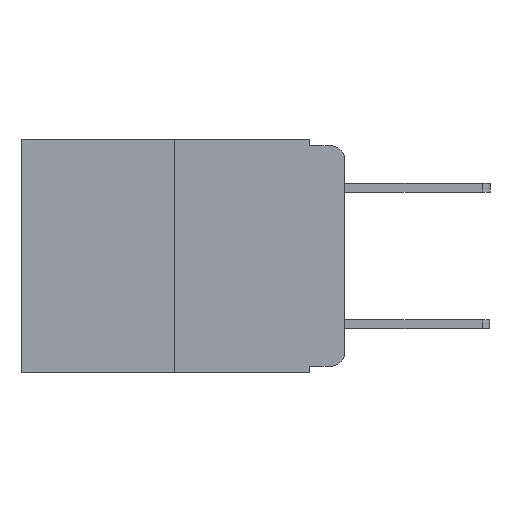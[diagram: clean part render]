
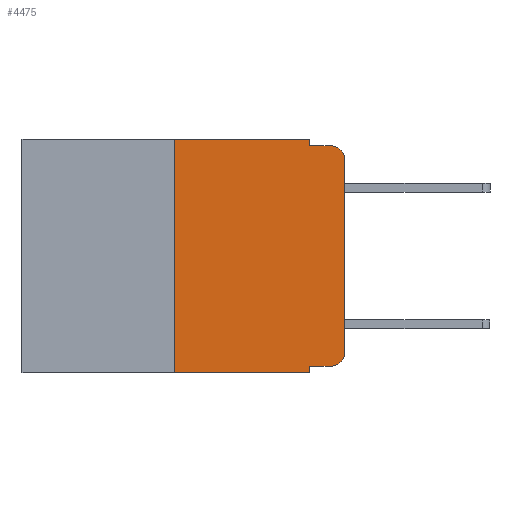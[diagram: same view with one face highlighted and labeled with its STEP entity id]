
A CAD part, left-side view. The second image highlights one B-rep face of the part: STEP entity #4475.
In plain terms, the highlighted planar face has unit normal (-1, 0, 0).
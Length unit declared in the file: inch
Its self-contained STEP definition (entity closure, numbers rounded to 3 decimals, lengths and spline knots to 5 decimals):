
#105 = DIRECTION ( 'NONE',  ( 0., -1., 0. ) ) ;
#121 = CARTESIAN_POINT ( 'NONE',  ( 0., 0., -0.03 ) ) ;
#200 = CARTESIAN_POINT ( 'NONE',  ( 0., 0.051, 0. ) ) ;
#212 = DIRECTION ( 'NONE',  ( 0., 0., -1. ) ) ;
#268 = EDGE_CURVE ( 'NONE', #2577, #10206, #4773, .T. ) ;
#276 = VECTOR ( 'NONE', #105, 39.37008 ) ;
#419 = CARTESIAN_POINT ( 'NONE',  ( 0., 0., -0.313 ) ) ;
#527 = CARTESIAN_POINT ( 'NONE',  ( 0., 0.051, -0.01 ) ) ;
#623 = VERTEX_POINT ( 'NONE', #8739 ) ;
#753 = EDGE_CURVE ( 'NONE', #2899, #10206, #7010, .T. ) ;
#766 = AXIS2_PLACEMENT_3D ( 'NONE', #10190, #7118, #7107 ) ;
#990 = DIRECTION ( 'NONE',  ( 0., 0., -1. ) ) ;
#1369 = EDGE_CURVE ( 'NONE', #623, #10590, #6262, .T. ) ;
#1704 = FACE_OUTER_BOUND ( 'NONE', #3279, .T. ) ;
#1706 = CARTESIAN_POINT ( 'NONE',  ( 0., 0.051, -0.333 ) ) ;
#1710 = EDGE_CURVE ( 'NONE', #2424, #2982, #9359, .T. ) ;
#2424 = VERTEX_POINT ( 'NONE', #121 ) ;
#2572 = ORIENTED_EDGE ( 'NONE', *, *, #1710, .T. ) ;
#2577 = VERTEX_POINT ( 'NONE', #7646 ) ;
#2582 = LINE ( 'NONE', #3655, #9008 ) ;
#2667 = ORIENTED_EDGE ( 'NONE', *, *, #1369, .T. ) ;
#2899 = VERTEX_POINT ( 'NONE', #8950 ) ;
#2982 = VERTEX_POINT ( 'NONE', #9451 ) ;
#3067 = CARTESIAN_POINT ( 'NONE',  ( 0., 0.051, -0.343 ) ) ;
#3092 = AXIS2_PLACEMENT_3D ( 'NONE', #5135, #5131, #5120 ) ;
#3255 = ORIENTED_EDGE ( 'NONE', *, *, #4224, .F. ) ;
#3279 = EDGE_LOOP ( 'NONE', ( #5029, #2572, #3952, #9219, #3255, #6819, #7959, #10661, #6292, #2667 ) ) ;
#3638 = VERTEX_POINT ( 'NONE', #9379 ) ;
#3655 = CARTESIAN_POINT ( 'NONE',  ( 0., 0.051, 0. ) ) ;
#3799 = EDGE_CURVE ( 'NONE', #10590, #2424, #4610, .T. ) ;
#3952 = ORIENTED_EDGE ( 'NONE', *, *, #10693, .F. ) ;
#4224 = EDGE_CURVE ( 'NONE', #9430, #9371, #9041, .T. ) ;
#4347 = VECTOR ( 'NONE', #9691, 39.37008 ) ;
#4475 = ADVANCED_FACE ( 'NONE', ( #1704 ), #5142, .F. ) ;
#4610 = LINE ( 'NONE', #9733, #4347 ) ;
#4732 = DIRECTION ( 'NONE',  ( 0., -1., 0. ) ) ;
#4773 = LINE ( 'NONE', #200, #8949 ) ;
#4891 = DIRECTION ( 'NONE',  ( 0., -1., 0. ) ) ;
#4912 = CARTESIAN_POINT ( 'NONE',  ( 0., 0.473, 0. ) ) ;
#5029 = ORIENTED_EDGE ( 'NONE', *, *, #3799, .T. ) ;
#5055 = CARTESIAN_POINT ( 'NONE',  ( 0., 0.25, 0. ) ) ;
#5120 = DIRECTION ( 'NONE',  ( 0., 0., -1. ) ) ;
#5131 = DIRECTION ( 'NONE',  ( 1., 0., 0. ) ) ;
#5135 = CARTESIAN_POINT ( 'NONE',  ( 0., 0.473, 0. ) ) ;
#5142 = PLANE ( 'NONE',  #3092 ) ;
#5366 = VECTOR ( 'NONE', #4732, 39.37008 ) ;
#5530 = EDGE_CURVE ( 'NONE', #9371, #3638, #2582, .T. ) ;
#5894 = LINE ( 'NONE', #527, #5366 ) ;
#6084 = VECTOR ( 'NONE', #10846, 39.37008 ) ;
#6262 = CIRCLE ( 'NONE', #10133, 0.02 ) ;
#6292 = ORIENTED_EDGE ( 'NONE', *, *, #7998, .T. ) ;
#6672 = DIRECTION ( 'NONE',  ( 0., 0., -1. ) ) ;
#6819 = ORIENTED_EDGE ( 'NONE', *, *, #7972, .F. ) ;
#6978 = CARTESIAN_POINT ( 'NONE',  ( 0., 0.051, 0. ) ) ;
#7010 = LINE ( 'NONE', #7906, #276 ) ;
#7107 = DIRECTION ( 'NONE',  ( 0., 0., -1. ) ) ;
#7118 = DIRECTION ( 'NONE',  ( -1., 0., 0. ) ) ;
#7556 = DIRECTION ( 'NONE',  ( 0., -1., 0. ) ) ;
#7646 = CARTESIAN_POINT ( 'NONE',  ( 0., 0.051, -0.333 ) ) ;
#7906 = CARTESIAN_POINT ( 'NONE',  ( 0., 0.473, -0.343 ) ) ;
#7959 = ORIENTED_EDGE ( 'NONE', *, *, #753, .T. ) ;
#7972 = EDGE_CURVE ( 'NONE', #2899, #9430, #10197, .T. ) ;
#7984 = LINE ( 'NONE', #1706, #10455 ) ;
#7998 = EDGE_CURVE ( 'NONE', #2577, #623, #7984, .T. ) ;
#8739 = CARTESIAN_POINT ( 'NONE',  ( 0., 0.02, -0.333 ) ) ;
#8784 = VECTOR ( 'NONE', #4891, 39.37008 ) ;
#8949 = VECTOR ( 'NONE', #212, 39.37008 ) ;
#8950 = CARTESIAN_POINT ( 'NONE',  ( 0., 0.25, -0.343 ) ) ;
#9008 = VECTOR ( 'NONE', #6672, 39.37008 ) ;
#9041 = LINE ( 'NONE', #4912, #8784 ) ;
#9219 = ORIENTED_EDGE ( 'NONE', *, *, #5530, .F. ) ;
#9359 = CIRCLE ( 'NONE', #766, 0.02 ) ;
#9371 = VERTEX_POINT ( 'NONE', #6978 ) ;
#9379 = CARTESIAN_POINT ( 'NONE',  ( 0., 0.051, -0.01 ) ) ;
#9430 = VERTEX_POINT ( 'NONE', #9525 ) ;
#9451 = CARTESIAN_POINT ( 'NONE',  ( 0., 0.02, -0.01 ) ) ;
#9525 = CARTESIAN_POINT ( 'NONE',  ( 0., 0.25, 0. ) ) ;
#9691 = DIRECTION ( 'NONE',  ( 0., 0., 1. ) ) ;
#9733 = CARTESIAN_POINT ( 'NONE',  ( 0., 0., 0. ) ) ;
#9916 = DIRECTION ( 'NONE',  ( -1., 0., 0. ) ) ;
#9941 = CARTESIAN_POINT ( 'NONE',  ( 0., 0.02, -0.313 ) ) ;
#10133 = AXIS2_PLACEMENT_3D ( 'NONE', #9941, #9916, #990 ) ;
#10190 = CARTESIAN_POINT ( 'NONE',  ( 0., 0.02, -0.03 ) ) ;
#10197 = LINE ( 'NONE', #5055, #6084 ) ;
#10206 = VERTEX_POINT ( 'NONE', #3067 ) ;
#10455 = VECTOR ( 'NONE', #7556, 39.37008 ) ;
#10590 = VERTEX_POINT ( 'NONE', #419 ) ;
#10661 = ORIENTED_EDGE ( 'NONE', *, *, #268, .F. ) ;
#10693 = EDGE_CURVE ( 'NONE', #3638, #2982, #5894, .T. ) ;
#10846 = DIRECTION ( 'NONE',  ( 0., 0., 1. ) ) ;
